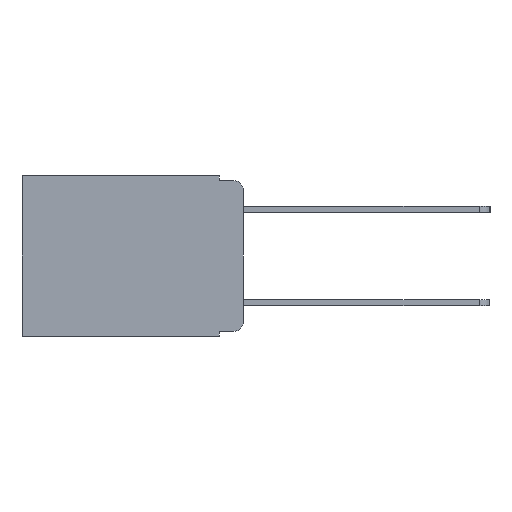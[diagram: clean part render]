
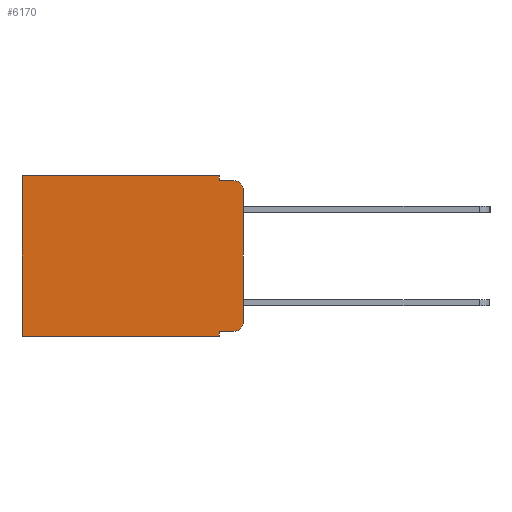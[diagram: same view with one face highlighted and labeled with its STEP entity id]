
A CAD part, left-side view. The second image highlights one B-rep face of the part: STEP entity #6170.
In plain terms, the highlighted planar face has unit normal (-1, 0, 0).
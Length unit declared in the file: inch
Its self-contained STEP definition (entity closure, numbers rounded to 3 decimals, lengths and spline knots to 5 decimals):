
#274 = EDGE_CURVE ( 'NONE', #7042, #3804, #9169, .T. ) ;
#790 = CARTESIAN_POINT ( 'NONE',  ( 0.298, 0.02, -0.313 ) ) ;
#856 = CARTESIAN_POINT ( 'NONE',  ( 0.298, 0., 0. ) ) ;
#935 = VECTOR ( 'NONE', #13371, 39.37008 ) ;
#993 = EDGE_CURVE ( 'NONE', #7042, #4924, #11479, .T. ) ;
#1008 = CIRCLE ( 'NONE', #11583, 0.02 ) ;
#1058 = VECTOR ( 'NONE', #11454, 39.37008 ) ;
#1226 = ORIENTED_EDGE ( 'NONE', *, *, #2347, .T. ) ;
#1568 = ORIENTED_EDGE ( 'NONE', *, *, #13649, .T. ) ;
#1710 = CARTESIAN_POINT ( 'NONE',  ( 0.298, 0.051, -0.01 ) ) ;
#2015 = CARTESIAN_POINT ( 'NONE',  ( 0.298, 0.051, 0. ) ) ;
#2158 = DIRECTION ( 'NONE',  ( 0., 0., -1. ) ) ;
#2238 = CARTESIAN_POINT ( 'NONE',  ( 0.298, 0., 0. ) ) ;
#2347 = EDGE_CURVE ( 'NONE', #9689, #4707, #12087, .T. ) ;
#2753 = LINE ( 'NONE', #856, #14155 ) ;
#2906 = EDGE_CURVE ( 'NONE', #3245, #9592, #14141, .T. ) ;
#3026 = LINE ( 'NONE', #10381, #5742 ) ;
#3034 = VECTOR ( 'NONE', #6518, 39.37008 ) ;
#3245 = VERTEX_POINT ( 'NONE', #3636 ) ;
#3572 = CARTESIAN_POINT ( 'NONE',  ( 0.298, 0., 0. ) ) ;
#3575 = DIRECTION ( 'NONE',  ( 0., 0., -1. ) ) ;
#3636 = CARTESIAN_POINT ( 'NONE',  ( 0.298, 0.051, 0. ) ) ;
#3694 = EDGE_CURVE ( 'NONE', #9592, #3804, #13664, .T. ) ;
#3804 = VERTEX_POINT ( 'NONE', #8885 ) ;
#4004 = CARTESIAN_POINT ( 'NONE',  ( 0.298, 0.02, -0.03 ) ) ;
#4327 = LINE ( 'NONE', #2015, #1058 ) ;
#4637 = ORIENTED_EDGE ( 'NONE', *, *, #3694, .F. ) ;
#4641 = VERTEX_POINT ( 'NONE', #5065 ) ;
#4707 = VERTEX_POINT ( 'NONE', #7948 ) ;
#4924 = VERTEX_POINT ( 'NONE', #9265 ) ;
#5063 = CARTESIAN_POINT ( 'NONE',  ( 0.298, 0.02, -0.333 ) ) ;
#5065 = CARTESIAN_POINT ( 'NONE',  ( 0.298, 0.051, -0.343 ) ) ;
#5095 = DIRECTION ( 'NONE',  ( 0., 1., 0. ) ) ;
#5195 = AXIS2_PLACEMENT_3D ( 'NONE', #2238, #6829, #14082 ) ;
#5276 = EDGE_CURVE ( 'NONE', #9230, #4641, #4327, .T. ) ;
#5730 = ORIENTED_EDGE ( 'NONE', *, *, #5276, .F. ) ;
#5742 = VECTOR ( 'NONE', #5095, 39.37008 ) ;
#5952 = CARTESIAN_POINT ( 'NONE',  ( 0.298, 0.051, -0.01 ) ) ;
#6101 = LINE ( 'NONE', #13798, #3034 ) ;
#6148 = DIRECTION ( 'NONE',  ( 0., 0., -1. ) ) ;
#6170 = ADVANCED_FACE ( 'NONE', ( #11222 ), #10967, .F. ) ;
#6518 = DIRECTION ( 'NONE',  ( 0., -1., 0. ) ) ;
#6651 = DIRECTION ( 'NONE',  ( 0., -1., 0. ) ) ;
#6814 = CARTESIAN_POINT ( 'NONE',  ( 0.298, 0.473, 0. ) ) ;
#6829 = DIRECTION ( 'NONE',  ( 1., 0., 0. ) ) ;
#6867 = CARTESIAN_POINT ( 'NONE',  ( 0.298, 0.051, 0. ) ) ;
#7042 = VERTEX_POINT ( 'NONE', #8056 ) ;
#7712 = ORIENTED_EDGE ( 'NONE', *, *, #8342, .T. ) ;
#7768 = DIRECTION ( 'NONE',  ( 0., 1., 0. ) ) ;
#7948 = CARTESIAN_POINT ( 'NONE',  ( 0.298, 0.473, -0.343 ) ) ;
#8056 = CARTESIAN_POINT ( 'NONE',  ( 0.298, 0., -0.03 ) ) ;
#8133 = VERTEX_POINT ( 'NONE', #5063 ) ;
#8342 = EDGE_CURVE ( 'NONE', #9230, #8133, #6101, .T. ) ;
#8398 = VECTOR ( 'NONE', #3575, 39.37008 ) ;
#8797 = EDGE_CURVE ( 'NONE', #4641, #4707, #3026, .T. ) ;
#8846 = DIRECTION ( 'NONE',  ( -1., 0., 0. ) ) ;
#8885 = CARTESIAN_POINT ( 'NONE',  ( 0.298, 0.02, -0.01 ) ) ;
#9169 = CIRCLE ( 'NONE', #10864, 0.02 ) ;
#9230 = VERTEX_POINT ( 'NONE', #10831 ) ;
#9265 = CARTESIAN_POINT ( 'NONE',  ( 0.298, 0., -0.313 ) ) ;
#9292 = ORIENTED_EDGE ( 'NONE', *, *, #2906, .F. ) ;
#9477 = DIRECTION ( 'NONE',  ( 0., 0., -1. ) ) ;
#9592 = VERTEX_POINT ( 'NONE', #1710 ) ;
#9689 = VERTEX_POINT ( 'NONE', #9835 ) ;
#9740 = EDGE_CURVE ( 'NONE', #8133, #4924, #1008, .T. ) ;
#9835 = CARTESIAN_POINT ( 'NONE',  ( 0.298, 0.473, 0. ) ) ;
#10381 = CARTESIAN_POINT ( 'NONE',  ( 0.298, 0., -0.343 ) ) ;
#10400 = ORIENTED_EDGE ( 'NONE', *, *, #993, .F. ) ;
#10749 = ORIENTED_EDGE ( 'NONE', *, *, #8797, .F. ) ;
#10831 = CARTESIAN_POINT ( 'NONE',  ( 0.298, 0.051, -0.333 ) ) ;
#10864 = AXIS2_PLACEMENT_3D ( 'NONE', #4004, #11570, #9477 ) ;
#10883 = VECTOR ( 'NONE', #6651, 39.37008 ) ;
#10967 = PLANE ( 'NONE',  #5195 ) ;
#11222 = FACE_OUTER_BOUND ( 'NONE', #11624, .T. ) ;
#11410 = VECTOR ( 'NONE', #6148, 39.37008 ) ;
#11454 = DIRECTION ( 'NONE',  ( 0., 0., -1. ) ) ;
#11479 = LINE ( 'NONE', #3572, #8398 ) ;
#11570 = DIRECTION ( 'NONE',  ( -1., 0., 0. ) ) ;
#11583 = AXIS2_PLACEMENT_3D ( 'NONE', #790, #8846, #2158 ) ;
#11624 = EDGE_LOOP ( 'NONE', ( #10400, #14418, #4637, #9292, #1568, #1226, #10749, #5730, #7712, #11997 ) ) ;
#11997 = ORIENTED_EDGE ( 'NONE', *, *, #9740, .T. ) ;
#12087 = LINE ( 'NONE', #6814, #935 ) ;
#13371 = DIRECTION ( 'NONE',  ( 0., 0., -1. ) ) ;
#13649 = EDGE_CURVE ( 'NONE', #3245, #9689, #2753, .T. ) ;
#13664 = LINE ( 'NONE', #5952, #10883 ) ;
#13798 = CARTESIAN_POINT ( 'NONE',  ( 0.298, 0.051, -0.333 ) ) ;
#14082 = DIRECTION ( 'NONE',  ( 0., 0., -1. ) ) ;
#14141 = LINE ( 'NONE', #6867, #11410 ) ;
#14155 = VECTOR ( 'NONE', #7768, 39.37008 ) ;
#14418 = ORIENTED_EDGE ( 'NONE', *, *, #274, .T. ) ;
